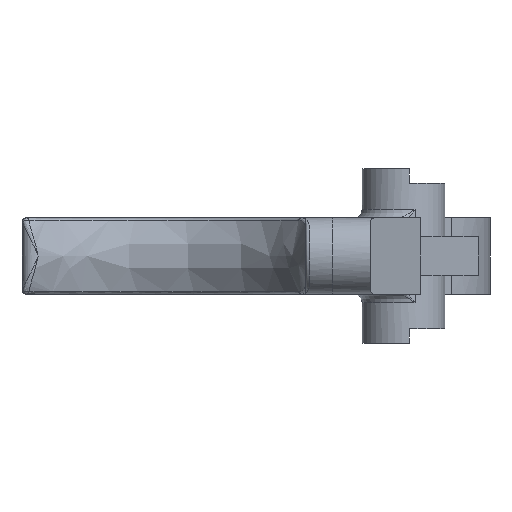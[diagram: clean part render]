
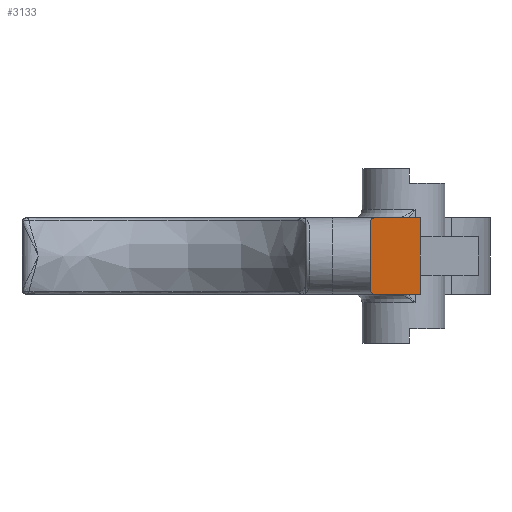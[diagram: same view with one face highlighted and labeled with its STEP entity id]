
A CAD part, left-side view. The second image highlights one B-rep face of the part: STEP entity #3133.
In plain terms, the highlighted planar face has unit normal (-0.99, 0.139, 0).
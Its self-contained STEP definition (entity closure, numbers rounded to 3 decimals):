
#22=ELLIPSE('',#3433,0.4,0.396);
#23=ELLIPSE('',#3434,0.4,0.396);
#235=FACE_OUTER_BOUND('',#419,.T.);
#419=EDGE_LOOP('',(#2496,#2497,#2498,#2499,#2500,#2501));
#748=LINE('',#6879,#942);
#792=LINE('',#7013,#986);
#812=LINE('',#12180,#1006);
#817=LINE('',#12210,#1011);
#942=VECTOR('',#3868,1000.);
#986=VECTOR('',#3958,1000.);
#1006=VECTOR('',#4050,1000.);
#1011=VECTOR('',#4065,1000.);
#1301=VERTEX_POINT('',#6876);
#1302=VERTEX_POINT('',#6878);
#1360=VERTEX_POINT('',#7010);
#1361=VERTEX_POINT('',#7012);
#1416=VERTEX_POINT('',#12208);
#1417=VERTEX_POINT('',#12209);
#1672=EDGE_CURVE('',#1301,#1302,#748,.T.);
#1738=EDGE_CURVE('',#1360,#1361,#792,.T.);
#1803=EDGE_CURVE('',#1302,#1360,#812,.T.);
#1813=EDGE_CURVE('',#1416,#1417,#817,.T.);
#1814=EDGE_CURVE('',#1417,#1361,#22,.T.);
#1815=EDGE_CURVE('',#1301,#1416,#23,.T.);
#2496=ORIENTED_EDGE('',*,*,#1813,.T.);
#2497=ORIENTED_EDGE('',*,*,#1814,.T.);
#2498=ORIENTED_EDGE('',*,*,#1738,.F.);
#2499=ORIENTED_EDGE('',*,*,#1803,.F.);
#2500=ORIENTED_EDGE('',*,*,#1672,.F.);
#2501=ORIENTED_EDGE('',*,*,#1815,.T.);
#3008=PLANE('',#3432);
#3133=ADVANCED_FACE('',(#235),#3008,.F.);
#3432=AXIS2_PLACEMENT_3D('',#12207,#4063,#4064);
#3433=AXIS2_PLACEMENT_3D('',#12211,#4066,#4067);
#3434=AXIS2_PLACEMENT_3D('',#12212,#4068,#4069);
#3868=DIRECTION('',(-0.139,-0.99,0.));
#3958=DIRECTION('',(0.139,0.99,0.));
#4050=DIRECTION('',(0.,0.,-1.));
#4063=DIRECTION('center_axis',(0.99,-0.139,0.));
#4064=DIRECTION('ref_axis',(0.,0.,-1.));
#4065=DIRECTION('',(0.,0.,-1.));
#4066=DIRECTION('center_axis',(-0.99,0.139,0.));
#4067=DIRECTION('ref_axis',(0.139,0.99,0.));
#4068=DIRECTION('center_axis',(-0.99,0.139,0.));
#4069=DIRECTION('ref_axis',(0.139,0.99,0.));
#6876=CARTESIAN_POINT('',(-10.756,-4.078,3.683));
#6878=CARTESIAN_POINT('',(-11.374,-8.476,3.683));
#6879=CARTESIAN_POINT('',(-10.756,-4.078,3.683));
#7010=CARTESIAN_POINT('',(-11.374,-8.476,-3.683));
#7012=CARTESIAN_POINT('',(-10.756,-4.078,-3.683));
#7013=CARTESIAN_POINT('',(-11.374,-8.476,-3.683));
#12180=CARTESIAN_POINT('',(-11.374,-8.476,3.683));
#12207=CARTESIAN_POINT('Origin',(-9.969,1.524,-7.468));
#12208=CARTESIAN_POINT('',(-10.7,-3.682,3.287));
#12209=CARTESIAN_POINT('',(-10.7,-3.682,-3.287));
#12210=CARTESIAN_POINT('',(-10.7,-3.682,3.287));
#12211=CARTESIAN_POINT('Origin',(-10.756,-4.078,-3.287));
#12212=CARTESIAN_POINT('Origin',(-10.756,-4.078,3.287));
